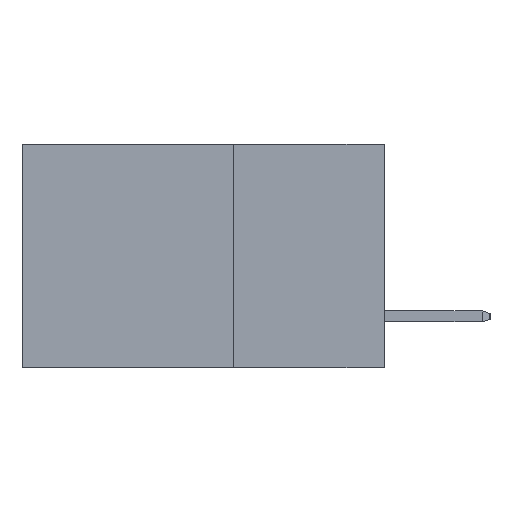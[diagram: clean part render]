
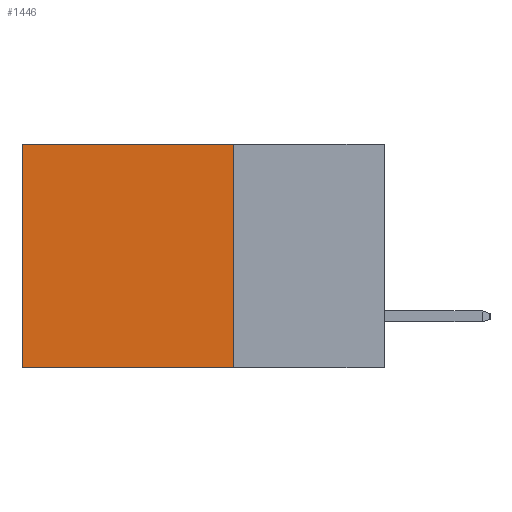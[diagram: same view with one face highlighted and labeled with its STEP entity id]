
A CAD part, left-side view. The second image highlights one B-rep face of the part: STEP entity #1446.
In plain terms, the highlighted planar face has unit normal (-1, 0, 0).
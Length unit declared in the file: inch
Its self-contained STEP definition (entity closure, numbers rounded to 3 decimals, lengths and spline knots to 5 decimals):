
#731 = LINE ( 'NONE', #26495, #5747 ) ;
#1446 = ADVANCED_FACE ( 'NONE', ( #27142 ), #2206, .F. ) ;
#2206 = PLANE ( 'NONE',  #26877 ) ;
#2278 = DIRECTION ( 'NONE',  ( 0., 0., -1. ) ) ;
#2529 = ORIENTED_EDGE ( 'NONE', *, *, #10418, .F. ) ;
#3718 = VERTEX_POINT ( 'NONE', #21480 ) ;
#4233 = ORIENTED_EDGE ( 'NONE', *, *, #16644, .T. ) ;
#4342 = LINE ( 'NONE', #8652, #16674 ) ;
#4926 = CARTESIAN_POINT ( 'NONE',  ( 0.298, 0.25, 0. ) ) ;
#5002 = VERTEX_POINT ( 'NONE', #14318 ) ;
#5747 = VECTOR ( 'NONE', #11690, 39.37008 ) ;
#8652 = CARTESIAN_POINT ( 'NONE',  ( 0.298, 0.25, 0. ) ) ;
#10418 = EDGE_CURVE ( 'NONE', #5002, #16113, #731, .T. ) ;
#11146 = DIRECTION ( 'NONE',  ( 0., 1., 0. ) ) ;
#11657 = ORIENTED_EDGE ( 'NONE', *, *, #16792, .T. ) ;
#11690 = DIRECTION ( 'NONE',  ( 0., 0., -1. ) ) ;
#12385 = EDGE_CURVE ( 'NONE', #16113, #24253, #23070, .T. ) ;
#13770 = CARTESIAN_POINT ( 'NONE',  ( 0.298, 0.25, -0.37 ) ) ;
#14318 = CARTESIAN_POINT ( 'NONE',  ( 0.298, 0.25, 0. ) ) ;
#16113 = VERTEX_POINT ( 'NONE', #13770 ) ;
#16583 = CARTESIAN_POINT ( 'NONE',  ( 0.298, 0.6, 0. ) ) ;
#16644 = EDGE_CURVE ( 'NONE', #5002, #3718, #4342, .T. ) ;
#16674 = VECTOR ( 'NONE', #11146, 39.37008 ) ;
#16792 = EDGE_CURVE ( 'NONE', #3718, #24253, #30837, .T. ) ;
#16991 = ORIENTED_EDGE ( 'NONE', *, *, #12385, .F. ) ;
#17807 = VECTOR ( 'NONE', #28950, 39.37008 ) ;
#19502 = DIRECTION ( 'NONE',  ( 0., 1., 0. ) ) ;
#21480 = CARTESIAN_POINT ( 'NONE',  ( 0.298, 0.6, 0. ) ) ;
#21500 = VECTOR ( 'NONE', #19502, 39.37008 ) ;
#22130 = CARTESIAN_POINT ( 'NONE',  ( 0.298, 0.6, -0.37 ) ) ;
#23070 = LINE ( 'NONE', #31727, #21500 ) ;
#24253 = VERTEX_POINT ( 'NONE', #22130 ) ;
#26495 = CARTESIAN_POINT ( 'NONE',  ( 0.298, 0.25, 0. ) ) ;
#26877 = AXIS2_PLACEMENT_3D ( 'NONE', #4926, #30500, #2278 ) ;
#27142 = FACE_OUTER_BOUND ( 'NONE', #31853, .T. ) ;
#28950 = DIRECTION ( 'NONE',  ( 0., 0., -1. ) ) ;
#30500 = DIRECTION ( 'NONE',  ( 1., 0., 0. ) ) ;
#30837 = LINE ( 'NONE', #16583, #17807 ) ;
#31727 = CARTESIAN_POINT ( 'NONE',  ( 0.298, 0.25, -0.37 ) ) ;
#31853 = EDGE_LOOP ( 'NONE', ( #11657, #16991, #2529, #4233 ) ) ;
